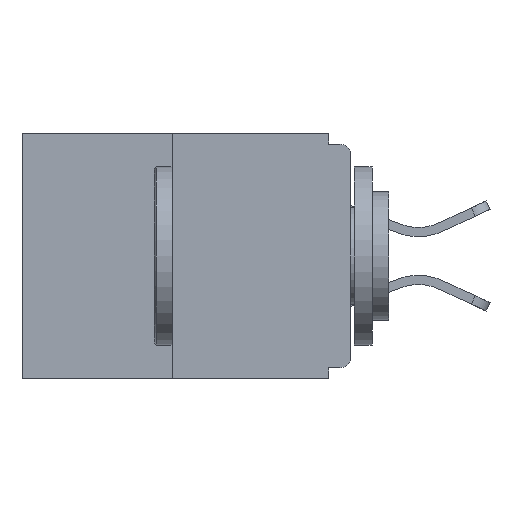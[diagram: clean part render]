
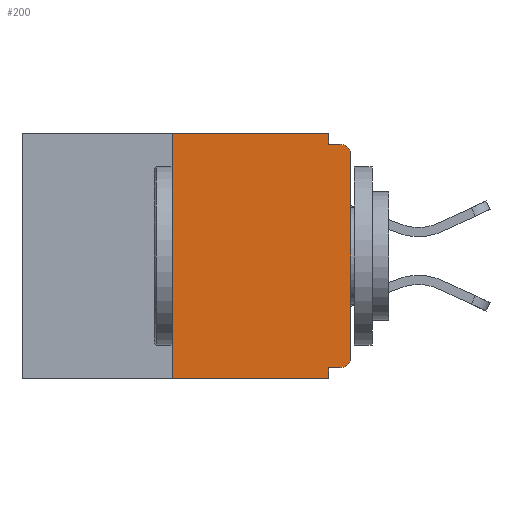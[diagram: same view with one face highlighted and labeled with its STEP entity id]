
A CAD part, left-side view. The second image highlights one B-rep face of the part: STEP entity #200.
In plain terms, the highlighted planar face has unit normal (-1, 0, 0).
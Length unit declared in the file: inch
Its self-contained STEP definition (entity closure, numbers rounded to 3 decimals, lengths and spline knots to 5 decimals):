
#200 = ADVANCED_FACE ( 'NONE', ( #11096 ), #5876, .F. ) ;
#245 = VECTOR ( 'NONE', #5679, 39.37008 ) ;
#1458 = CARTESIAN_POINT ( 'NONE',  ( 0., 0.46, 0. ) ) ;
#1510 = VERTEX_POINT ( 'NONE', #6918 ) ;
#1719 = ORIENTED_EDGE ( 'NONE', *, *, #14771, .F. ) ;
#1748 = CARTESIAN_POINT ( 'NONE',  ( 0., 0.46, -0.343 ) ) ;
#2096 = CARTESIAN_POINT ( 'NONE',  ( 0., 0.25, 0. ) ) ;
#2145 = VERTEX_POINT ( 'NONE', #7729 ) ;
#2411 = LINE ( 'NONE', #1748, #9705 ) ;
#2582 = DIRECTION ( 'NONE',  ( -1., 0., 0. ) ) ;
#2944 = VERTEX_POINT ( 'NONE', #16953 ) ;
#3016 = CIRCLE ( 'NONE', #17462, 0.015 ) ;
#3050 = DIRECTION ( 'NONE',  ( -1., 0., 0. ) ) ;
#3159 = DIRECTION ( 'NONE',  ( 0., -1., 0. ) ) ;
#3198 = ORIENTED_EDGE ( 'NONE', *, *, #10196, .F. ) ;
#3332 = EDGE_LOOP ( 'NONE', ( #1719, #13955, #11839, #3198, #14667, #10204, #16096, #13523, #4180, #5964 ) ) ;
#3646 = VERTEX_POINT ( 'NONE', #15504 ) ;
#3672 = CARTESIAN_POINT ( 'NONE',  ( 0., 0.015, -0.015 ) ) ;
#3742 = DIRECTION ( 'NONE',  ( 0., 0., -1. ) ) ;
#3980 = CARTESIAN_POINT ( 'NONE',  ( 0., 0.25, -0.343 ) ) ;
#3997 = VECTOR ( 'NONE', #14075, 39.37008 ) ;
#4158 = LINE ( 'NONE', #5490, #245 ) ;
#4180 = ORIENTED_EDGE ( 'NONE', *, *, #12689, .F. ) ;
#4714 = DIRECTION ( 'NONE',  ( 0., -1., 0. ) ) ;
#5245 = LINE ( 'NONE', #17922, #7059 ) ;
#5485 = EDGE_CURVE ( 'NONE', #2944, #17591, #3016, .T. ) ;
#5490 = CARTESIAN_POINT ( 'NONE',  ( 0., 0., 0. ) ) ;
#5679 = DIRECTION ( 'NONE',  ( 0., 0., 1. ) ) ;
#5684 = VECTOR ( 'NONE', #4714, 39.37008 ) ;
#5873 = VERTEX_POINT ( 'NONE', #10433 ) ;
#5876 = PLANE ( 'NONE',  #8235 ) ;
#5964 = ORIENTED_EDGE ( 'NONE', *, *, #15004, .F. ) ;
#6129 = EDGE_CURVE ( 'NONE', #7415, #2145, #2411, .T. ) ;
#6152 = VERTEX_POINT ( 'NONE', #14876 ) ;
#6337 = VECTOR ( 'NONE', #16292, 39.37008 ) ;
#6396 = EDGE_CURVE ( 'NONE', #7415, #5873, #11048, .T. ) ;
#6504 = VECTOR ( 'NONE', #16537, 39.37008 ) ;
#6540 = VERTEX_POINT ( 'NONE', #12493 ) ;
#6816 = LINE ( 'NONE', #17849, #6337 ) ;
#6918 = CARTESIAN_POINT ( 'NONE',  ( 0., 0.031, 0. ) ) ;
#7059 = VECTOR ( 'NONE', #13469, 39.37008 ) ;
#7415 = VERTEX_POINT ( 'NONE', #3980 ) ;
#7660 = AXIS2_PLACEMENT_3D ( 'NONE', #10321, #3050, #14718 ) ;
#7729 = CARTESIAN_POINT ( 'NONE',  ( 0., 0.031, -0.343 ) ) ;
#7911 = DIRECTION ( 'NONE',  ( 0., 0., 1. ) ) ;
#8111 = VECTOR ( 'NONE', #7911, 39.37008 ) ;
#8235 = AXIS2_PLACEMENT_3D ( 'NONE', #1458, #10138, #16040 ) ;
#8355 = CARTESIAN_POINT ( 'NONE',  ( 0., 0.46, 0. ) ) ;
#9143 = VERTEX_POINT ( 'NONE', #3672 ) ;
#9705 = VECTOR ( 'NONE', #3159, 39.37008 ) ;
#10138 = DIRECTION ( 'NONE',  ( 1., 0., 0. ) ) ;
#10196 = EDGE_CURVE ( 'NONE', #3646, #2145, #6816, .T. ) ;
#10204 = ORIENTED_EDGE ( 'NONE', *, *, #5485, .T. ) ;
#10321 = CARTESIAN_POINT ( 'NONE',  ( 0., 0.015, -0.03 ) ) ;
#10433 = CARTESIAN_POINT ( 'NONE',  ( 0., 0.25, 0. ) ) ;
#10648 = CIRCLE ( 'NONE', #7660, 0.015 ) ;
#11048 = LINE ( 'NONE', #2096, #8111 ) ;
#11096 = FACE_OUTER_BOUND ( 'NONE', #3332, .T. ) ;
#11330 = EDGE_CURVE ( 'NONE', #6540, #9143, #10648, .T. ) ;
#11839 = ORIENTED_EDGE ( 'NONE', *, *, #6129, .T. ) ;
#12091 = CARTESIAN_POINT ( 'NONE',  ( 0., 0.031, 0. ) ) ;
#12291 = EDGE_CURVE ( 'NONE', #2944, #3646, #5245, .T. ) ;
#12493 = CARTESIAN_POINT ( 'NONE',  ( 0., 0., -0.03 ) ) ;
#12516 = CARTESIAN_POINT ( 'NONE',  ( 0., 0., -0.313 ) ) ;
#12689 = EDGE_CURVE ( 'NONE', #6152, #9143, #13656, .T. ) ;
#13439 = CARTESIAN_POINT ( 'NONE',  ( 0., 0., -0.015 ) ) ;
#13469 = DIRECTION ( 'NONE',  ( 0., 1., 0. ) ) ;
#13523 = ORIENTED_EDGE ( 'NONE', *, *, #11330, .T. ) ;
#13656 = LINE ( 'NONE', #13439, #5684 ) ;
#13955 = ORIENTED_EDGE ( 'NONE', *, *, #6396, .F. ) ;
#14075 = DIRECTION ( 'NONE',  ( 0., -1., 0. ) ) ;
#14667 = ORIENTED_EDGE ( 'NONE', *, *, #12291, .F. ) ;
#14715 = LINE ( 'NONE', #12091, #6504 ) ;
#14718 = DIRECTION ( 'NONE',  ( 0., 0., -1. ) ) ;
#14771 = EDGE_CURVE ( 'NONE', #5873, #1510, #15603, .T. ) ;
#14876 = CARTESIAN_POINT ( 'NONE',  ( 0., 0.031, -0.015 ) ) ;
#15004 = EDGE_CURVE ( 'NONE', #1510, #6152, #14715, .T. ) ;
#15504 = CARTESIAN_POINT ( 'NONE',  ( 0., 0.031, -0.328 ) ) ;
#15603 = LINE ( 'NONE', #8355, #3997 ) ;
#16040 = DIRECTION ( 'NONE',  ( 0., 0., -1. ) ) ;
#16096 = ORIENTED_EDGE ( 'NONE', *, *, #17726, .T. ) ;
#16292 = DIRECTION ( 'NONE',  ( 0., 0., -1. ) ) ;
#16537 = DIRECTION ( 'NONE',  ( 0., 0., -1. ) ) ;
#16953 = CARTESIAN_POINT ( 'NONE',  ( 0., 0.015, -0.328 ) ) ;
#17462 = AXIS2_PLACEMENT_3D ( 'NONE', #18562, #2582, #3742 ) ;
#17591 = VERTEX_POINT ( 'NONE', #12516 ) ;
#17726 = EDGE_CURVE ( 'NONE', #17591, #6540, #4158, .T. ) ;
#17849 = CARTESIAN_POINT ( 'NONE',  ( 0., 0.031, -0.343 ) ) ;
#17922 = CARTESIAN_POINT ( 'NONE',  ( 0., 0., -0.328 ) ) ;
#18562 = CARTESIAN_POINT ( 'NONE',  ( 0., 0.015, -0.313 ) ) ;
